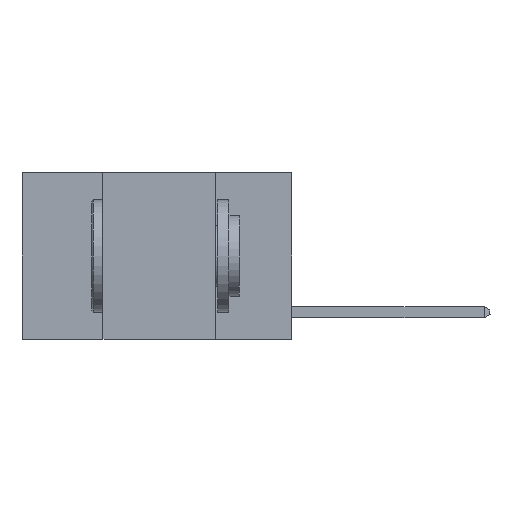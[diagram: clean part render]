
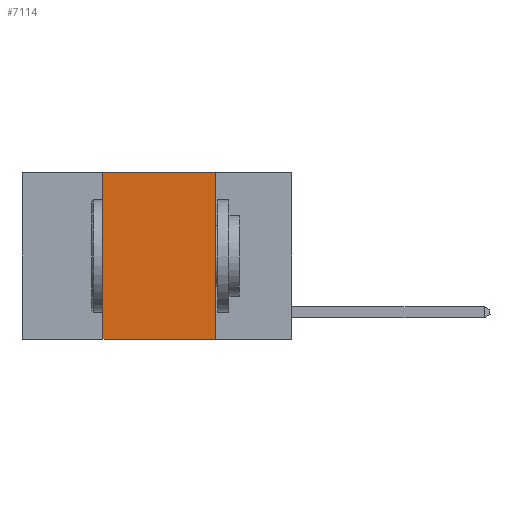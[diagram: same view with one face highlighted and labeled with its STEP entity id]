
A CAD part, left-side view. The second image highlights one B-rep face of the part: STEP entity #7114.
In plain terms, the highlighted planar face has unit normal (-1, 0, 0).
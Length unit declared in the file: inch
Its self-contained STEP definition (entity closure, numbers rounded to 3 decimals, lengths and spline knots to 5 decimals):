
#70 = LINE ( 'NONE', #9251, #6319 ) ;
#411 = CARTESIAN_POINT ( 'NONE',  ( 0., 0.42, -0.37 ) ) ;
#725 = CARTESIAN_POINT ( 'NONE',  ( 0., 0.42, 0. ) ) ;
#879 = CARTESIAN_POINT ( 'NONE',  ( 0., 0.17, 0. ) ) ;
#2066 = CARTESIAN_POINT ( 'NONE',  ( 0., 0.17, 0. ) ) ;
#2137 = DIRECTION ( 'NONE',  ( 0., -1., 0. ) ) ;
#2220 = DIRECTION ( 'NONE',  ( 1., 0., 0. ) ) ;
#2347 = DIRECTION ( 'NONE',  ( 0., 0., -1. ) ) ;
#2837 = LINE ( 'NONE', #8613, #4971 ) ;
#2958 = CARTESIAN_POINT ( 'NONE',  ( 0., 0.6, 0. ) ) ;
#3171 = LINE ( 'NONE', #879, #6247 ) ;
#3257 = CARTESIAN_POINT ( 'NONE',  ( 0., 0.6, 0. ) ) ;
#3454 = ORIENTED_EDGE ( 'NONE', *, *, #8182, .F. ) ;
#4276 = ORIENTED_EDGE ( 'NONE', *, *, #4617, .F. ) ;
#4573 = EDGE_CURVE ( 'NONE', #4621, #9752, #9639, .T. ) ;
#4617 = EDGE_CURVE ( 'NONE', #9752, #6050, #3171, .T. ) ;
#4621 = VERTEX_POINT ( 'NONE', #725 ) ;
#4971 = VECTOR ( 'NONE', #10366, 39.37008 ) ;
#5664 = ORIENTED_EDGE ( 'NONE', *, *, #9167, .T. ) ;
#6050 = VERTEX_POINT ( 'NONE', #10227 ) ;
#6126 = EDGE_LOOP ( 'NONE', ( #4276, #6548, #3454, #5664 ) ) ;
#6247 = VECTOR ( 'NONE', #2347, 39.37008 ) ;
#6319 = VECTOR ( 'NONE', #8478, 39.37008 ) ;
#6548 = ORIENTED_EDGE ( 'NONE', *, *, #4573, .F. ) ;
#6586 = DIRECTION ( 'NONE',  ( 0., 0., -1. ) ) ;
#7114 = ADVANCED_FACE ( 'NONE', ( #7262 ), #10743, .F. ) ;
#7262 = FACE_OUTER_BOUND ( 'NONE', #6126, .T. ) ;
#7799 = VERTEX_POINT ( 'NONE', #411 ) ;
#8182 = EDGE_CURVE ( 'NONE', #7799, #4621, #2837, .T. ) ;
#8478 = DIRECTION ( 'NONE',  ( 0., -1., 0. ) ) ;
#8613 = CARTESIAN_POINT ( 'NONE',  ( 0., 0.42, 0. ) ) ;
#8663 = AXIS2_PLACEMENT_3D ( 'NONE', #3257, #2220, #6586 ) ;
#9167 = EDGE_CURVE ( 'NONE', #7799, #6050, #70, .T. ) ;
#9251 = CARTESIAN_POINT ( 'NONE',  ( 0., 0.6, -0.37 ) ) ;
#9639 = LINE ( 'NONE', #2958, #9948 ) ;
#9752 = VERTEX_POINT ( 'NONE', #2066 ) ;
#9948 = VECTOR ( 'NONE', #2137, 39.37008 ) ;
#10227 = CARTESIAN_POINT ( 'NONE',  ( 0., 0.17, -0.37 ) ) ;
#10366 = DIRECTION ( 'NONE',  ( 0., 0., 1. ) ) ;
#10743 = PLANE ( 'NONE',  #8663 ) ;
